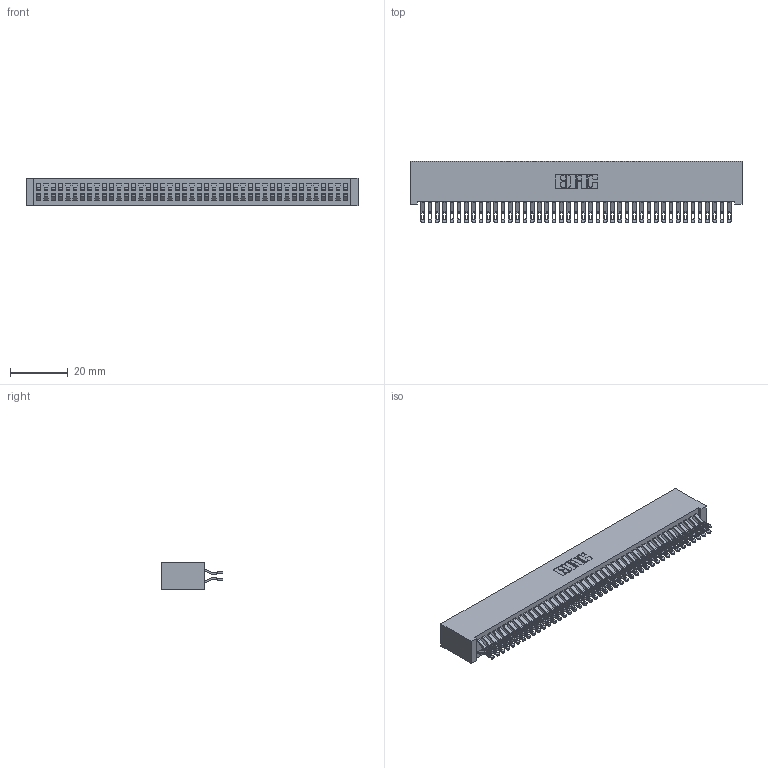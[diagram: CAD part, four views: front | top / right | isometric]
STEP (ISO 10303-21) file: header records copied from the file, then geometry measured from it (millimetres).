
FILE_DESCRIPTION (( 'STEP AP203' ), '1' );
FILE_NAME ('392-086-555-201.STEP', '2019-10-09T16:20:57', ( '' ), ( '' ), 'SwSTEP 2.0', 'SolidWorks 2016', '' );
FILE_SCHEMA (( 'CONFIG_CONTROL_DESIGN' ));
Length unit declared in the file: inch
Products named in the file (3): 392-086-555-201; 342 Part_Lugless; 345-292-001_555 Tail
Assembly tree (87 placements, depth 2):
  392-086-555-201
    342 Part_Lugless
    345-292-001_555 Tail  x86
Bounding box: 115.47 x 21.47 x 9.4 mm (x, y, z)
Volume: 11058.1 mm3; surface area: 19302.7 mm2
Topology: 87 solids, 87 shells, 5090 faces, 16013 edges, 10674 vertices
Faces by surface type: plane 2986, cylinder 2104
Entity records: 27451 total; most frequent: CARTESIAN_POINT 4580, ORIENTED_EDGE 4486, DIRECTION 3875, EDGE_CURVE 2243, VECTOR 2103, LINE 2103, VERTEX_POINT 1494, AXIS2_PLACEMENT_3D 886
